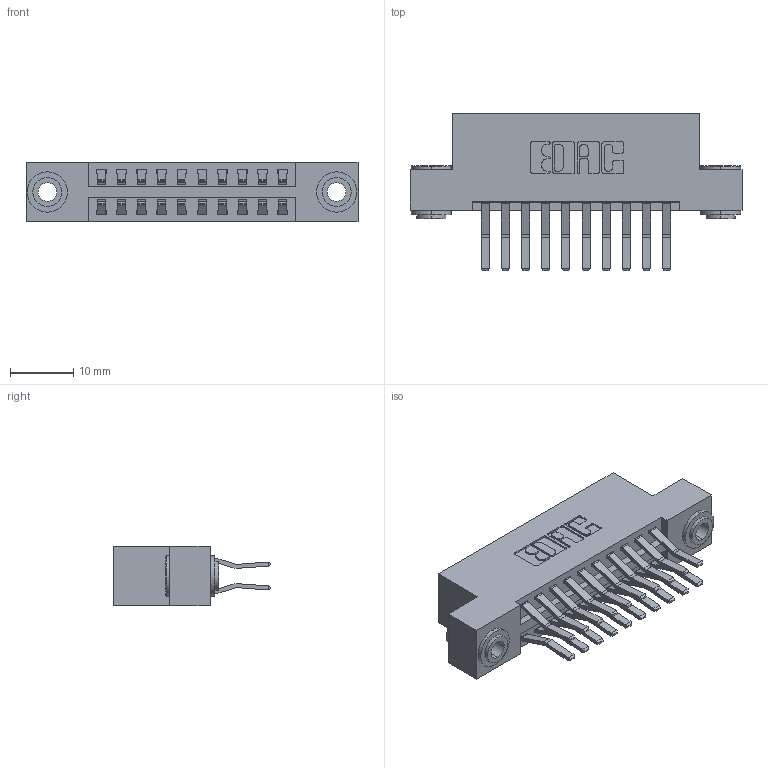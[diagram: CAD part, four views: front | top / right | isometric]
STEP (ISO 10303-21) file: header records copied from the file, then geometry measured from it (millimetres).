
FILE_DESCRIPTION (( 'STEP AP203' ), '1' );
FILE_NAME ('346-020-560-203.STEP', '2022-05-18T20:15:20', ( '' ), ( '' ), 'SwSTEP 2.0', 'SolidWorks 2020', '' );
FILE_SCHEMA (( 'CONFIG_CONTROL_DESIGN' ));
Length unit declared in the file: inch
Products named in the file (4): 345-292-001_560 Tail; 345-250-002_345-250-002-102; 346-020-560-203; 346 Part_Flush Mounting Lugs - 0.156 Dia-TH
Assembly tree (23 placements, depth 2):
  346-020-560-203
    346 Part_Flush Mounting Lugs - 0.156 Dia-TH
    345-292-001_560 Tail  x20
    345-250-002_345-250-002-102  x2
Bounding box: 52.32 x 24.78 x 9.4 mm (x, y, z)
Volume: 418.3 mm3; surface area: 6949.2 mm2
Topology: 22 solids, 23 shells, 1254 faces, 3661 edges, 2410 vertices
Faces by surface type: plane 800, cylinder 446, cone 8
Entity records: 11988 total; most frequent: CARTESIAN_POINT 2001, ORIENTED_EDGE 1926, DIRECTION 1849, EDGE_CURVE 963, VECTOR 763, LINE 763, VERTEX_POINT 638, AXIS2_PLACEMENT_3D 543
